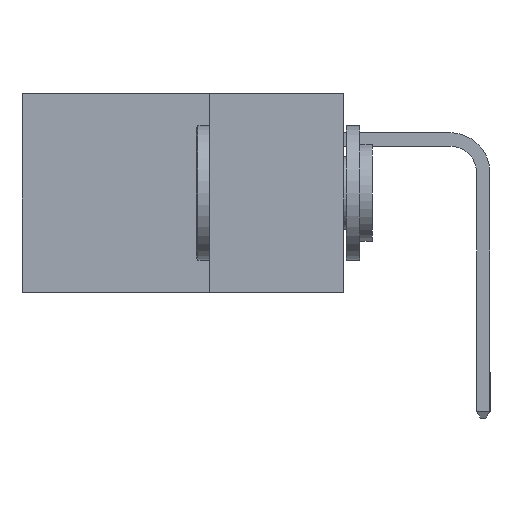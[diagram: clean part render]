
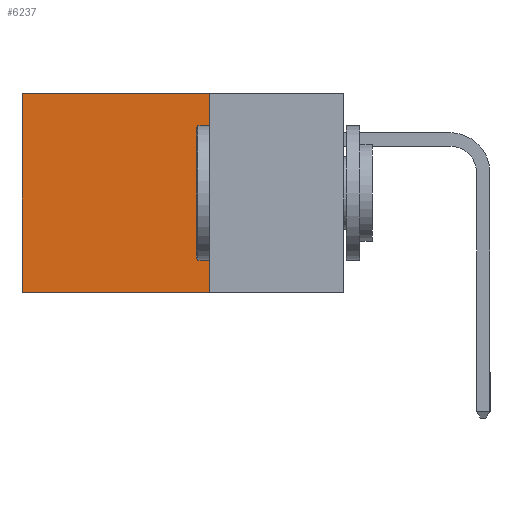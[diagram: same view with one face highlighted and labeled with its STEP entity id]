
A CAD part, left-side view. The second image highlights one B-rep face of the part: STEP entity #6237.
In plain terms, the highlighted planar face has unit normal (-1, 0, 0).
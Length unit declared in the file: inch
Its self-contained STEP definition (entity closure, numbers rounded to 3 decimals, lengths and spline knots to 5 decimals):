
#743 = EDGE_CURVE ( 'NONE', #18857, #9065, #5233, .T. ) ;
#1541 = PLANE ( 'NONE',  #2420 ) ;
#2420 = AXIS2_PLACEMENT_3D ( 'NONE', #18564, #10220, #15109 ) ;
#3112 = EDGE_CURVE ( 'NONE', #17206, #9065, #14925, .T. ) ;
#5233 = LINE ( 'NONE', #17295, #14040 ) ;
#5298 = EDGE_LOOP ( 'NONE', ( #20890, #12649, #15622, #10835 ) ) ;
#5387 = CARTESIAN_POINT ( 'NONE',  ( 0.298, 0.6, 0. ) ) ;
#6237 = ADVANCED_FACE ( 'NONE', ( #8564 ), #1541, .F. ) ;
#6515 = CARTESIAN_POINT ( 'NONE',  ( 0.298, 0.25, 0. ) ) ;
#6518 = VECTOR ( 'NONE', #10169, 39.37008 ) ;
#6569 = CARTESIAN_POINT ( 'NONE',  ( 0.298, 0.25, 0. ) ) ;
#6920 = CARTESIAN_POINT ( 'NONE',  ( 0.298, 0.25, 0. ) ) ;
#7482 = VECTOR ( 'NONE', #11581, 39.37008 ) ;
#8564 = FACE_OUTER_BOUND ( 'NONE', #5298, .T. ) ;
#9065 = VERTEX_POINT ( 'NONE', #10894 ) ;
#10169 = DIRECTION ( 'NONE',  ( 0., 0., -1. ) ) ;
#10220 = DIRECTION ( 'NONE',  ( 1., 0., 0. ) ) ;
#10835 = ORIENTED_EDGE ( 'NONE', *, *, #21067, .T. ) ;
#10894 = CARTESIAN_POINT ( 'NONE',  ( 0.298, 0.6, -0.37 ) ) ;
#11581 = DIRECTION ( 'NONE',  ( 0., 1., 0. ) ) ;
#12649 = ORIENTED_EDGE ( 'NONE', *, *, #3112, .F. ) ;
#14040 = VECTOR ( 'NONE', #19050, 39.37008 ) ;
#14338 = CARTESIAN_POINT ( 'NONE',  ( 0.298, 0.25, -0.37 ) ) ;
#14925 = LINE ( 'NONE', #21791, #7482 ) ;
#15109 = DIRECTION ( 'NONE',  ( 0., 0., -1. ) ) ;
#15622 = ORIENTED_EDGE ( 'NONE', *, *, #15830, .F. ) ;
#15830 = EDGE_CURVE ( 'NONE', #18100, #17206, #21247, .T. ) ;
#17206 = VERTEX_POINT ( 'NONE', #14338 ) ;
#17295 = CARTESIAN_POINT ( 'NONE',  ( 0.298, 0.6, 0. ) ) ;
#18085 = LINE ( 'NONE', #6515, #19420 ) ;
#18100 = VERTEX_POINT ( 'NONE', #6920 ) ;
#18564 = CARTESIAN_POINT ( 'NONE',  ( 0.298, 0.25, 0. ) ) ;
#18682 = DIRECTION ( 'NONE',  ( 0., 1., 0. ) ) ;
#18857 = VERTEX_POINT ( 'NONE', #5387 ) ;
#19050 = DIRECTION ( 'NONE',  ( 0., 0., -1. ) ) ;
#19420 = VECTOR ( 'NONE', #18682, 39.37008 ) ;
#20890 = ORIENTED_EDGE ( 'NONE', *, *, #743, .T. ) ;
#21067 = EDGE_CURVE ( 'NONE', #18100, #18857, #18085, .T. ) ;
#21247 = LINE ( 'NONE', #6569, #6518 ) ;
#21791 = CARTESIAN_POINT ( 'NONE',  ( 0.298, 0.25, -0.37 ) ) ;
